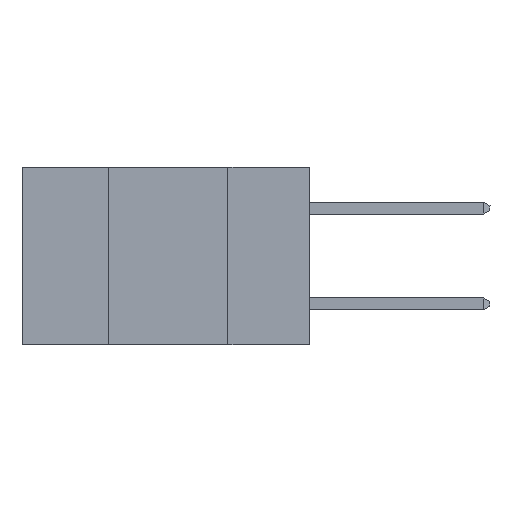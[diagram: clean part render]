
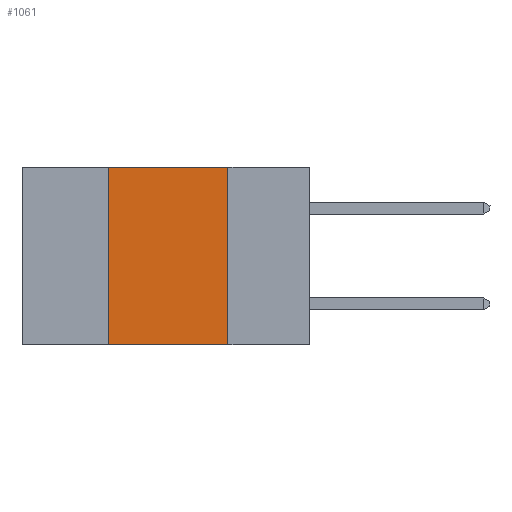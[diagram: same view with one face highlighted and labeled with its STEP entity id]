
A CAD part, left-side view. The second image highlights one B-rep face of the part: STEP entity #1061.
In plain terms, the highlighted planar face has unit normal (-1, 0, 0).
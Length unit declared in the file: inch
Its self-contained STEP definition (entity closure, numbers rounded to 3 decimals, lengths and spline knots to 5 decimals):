
#73 = VECTOR ( 'NONE', #576, 39.37008 ) ;
#576 = DIRECTION ( 'NONE',  ( 0., 0., 1. ) ) ;
#701 = EDGE_CURVE ( 'NONE', #6203, #880, #5742, .T. ) ;
#880 = VERTEX_POINT ( 'NONE', #7372 ) ;
#1061 = ADVANCED_FACE ( 'NONE', ( #6756 ), #10143, .F. ) ;
#1261 = VECTOR ( 'NONE', #3796, 39.37008 ) ;
#2332 = CARTESIAN_POINT ( 'NONE',  ( 0., 0.42, 0. ) ) ;
#2336 = CARTESIAN_POINT ( 'NONE',  ( 0., 0.17, 0. ) ) ;
#2765 = DIRECTION ( 'NONE',  ( 0., 0., -1. ) ) ;
#2920 = CARTESIAN_POINT ( 'NONE',  ( 0., 0.6, 0. ) ) ;
#3416 = VERTEX_POINT ( 'NONE', #2332 ) ;
#3430 = ORIENTED_EDGE ( 'NONE', *, *, #9408, .T. ) ;
#3667 = CARTESIAN_POINT ( 'NONE',  ( 0., 0.6, -0.37 ) ) ;
#3796 = DIRECTION ( 'NONE',  ( 0., -1., 0. ) ) ;
#4021 = VECTOR ( 'NONE', #6166, 39.37008 ) ;
#4124 = VERTEX_POINT ( 'NONE', #9682 ) ;
#4130 = ORIENTED_EDGE ( 'NONE', *, *, #5925, .F. ) ;
#4182 = AXIS2_PLACEMENT_3D ( 'NONE', #10541, #9885, #9818 ) ;
#4919 = ORIENTED_EDGE ( 'NONE', *, *, #701, .F. ) ;
#4933 = LINE ( 'NONE', #10633, #73 ) ;
#5742 = LINE ( 'NONE', #8985, #6009 ) ;
#5925 = EDGE_CURVE ( 'NONE', #3416, #6203, #5926, .T. ) ;
#5926 = LINE ( 'NONE', #2920, #1261 ) ;
#6009 = VECTOR ( 'NONE', #2765, 39.37008 ) ;
#6166 = DIRECTION ( 'NONE',  ( 0., -1., 0. ) ) ;
#6203 = VERTEX_POINT ( 'NONE', #2336 ) ;
#6383 = ORIENTED_EDGE ( 'NONE', *, *, #10463, .F. ) ;
#6756 = FACE_OUTER_BOUND ( 'NONE', #7128, .T. ) ;
#7128 = EDGE_LOOP ( 'NONE', ( #4919, #4130, #6383, #3430 ) ) ;
#7372 = CARTESIAN_POINT ( 'NONE',  ( 0., 0.17, -0.37 ) ) ;
#8985 = CARTESIAN_POINT ( 'NONE',  ( 0., 0.17, 0. ) ) ;
#9408 = EDGE_CURVE ( 'NONE', #4124, #880, #10409, .T. ) ;
#9682 = CARTESIAN_POINT ( 'NONE',  ( 0., 0.42, -0.37 ) ) ;
#9818 = DIRECTION ( 'NONE',  ( 0., 0., -1. ) ) ;
#9885 = DIRECTION ( 'NONE',  ( 1., 0., 0. ) ) ;
#10143 = PLANE ( 'NONE',  #4182 ) ;
#10409 = LINE ( 'NONE', #3667, #4021 ) ;
#10463 = EDGE_CURVE ( 'NONE', #4124, #3416, #4933, .T. ) ;
#10541 = CARTESIAN_POINT ( 'NONE',  ( 0., 0.6, 0. ) ) ;
#10633 = CARTESIAN_POINT ( 'NONE',  ( 0., 0.42, 0. ) ) ;
